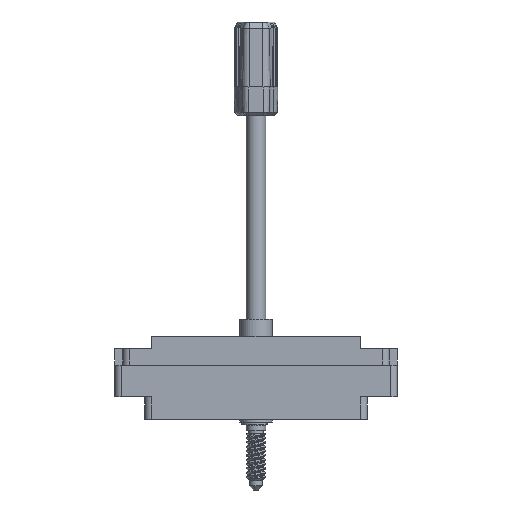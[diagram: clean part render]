
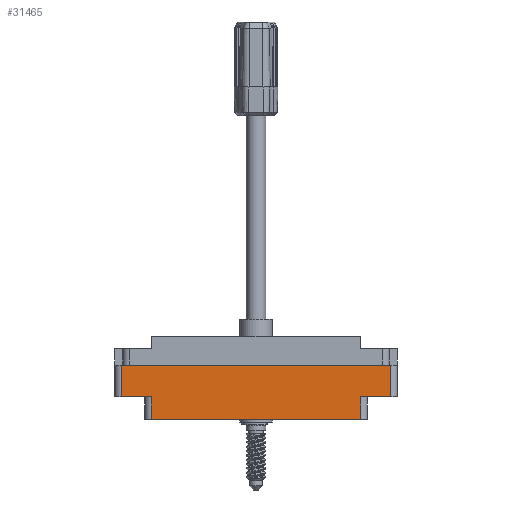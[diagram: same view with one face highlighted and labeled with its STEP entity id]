
A CAD part, front view. The second image highlights one B-rep face of the part: STEP entity #31465.
In plain terms, the highlighted planar face has unit normal (0, -1, 0).
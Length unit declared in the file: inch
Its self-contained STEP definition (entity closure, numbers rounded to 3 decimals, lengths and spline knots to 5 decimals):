
#426 = VERTEX_POINT ( 'NONE', #4976 ) ;
#4279 = VERTEX_POINT ( 'NONE', #10508 ) ;
#4976 = CARTESIAN_POINT ( 'NONE',  ( -1.297, -0.617, -0.274 ) ) ;
#5175 = VERTEX_POINT ( 'NONE', #20055 ) ;
#5830 = EDGE_CURVE ( 'NONE', #5175, #44853, #7103, .T. ) ;
#6219 = EDGE_CURVE ( 'NONE', #52509, #16943, #56597, .T. ) ;
#7103 = LINE ( 'NONE', #20857, #74675 ) ;
#7505 = EDGE_CURVE ( 'NONE', #44853, #25345, #31571, .T. ) ;
#8414 = LINE ( 'NONE', #32848, #31123 ) ;
#8819 = DIRECTION ( 'NONE',  ( 1., 0., 0. ) ) ;
#10450 = ORIENTED_EDGE ( 'NONE', *, *, #16627, .T. ) ;
#10508 = CARTESIAN_POINT ( 'NONE',  ( 1.006, -0.617, -0.798 ) ) ;
#11033 = CARTESIAN_POINT ( 'NONE',  ( -1.006, -0.617, -0.798 ) ) ;
#12350 = VERTEX_POINT ( 'NONE', #67529 ) ;
#12927 = AXIS2_PLACEMENT_3D ( 'NONE', #25637, #32825, #50704 ) ;
#14526 = EDGE_CURVE ( 'NONE', #426, #5175, #35365, .T. ) ;
#15360 = VECTOR ( 'NONE', #67457, 39.37008 ) ;
#16224 = DIRECTION ( 'NONE',  ( -1., 0., 0. ) ) ;
#16627 = EDGE_CURVE ( 'NONE', #52509, #12350, #61151, .T. ) ;
#16943 = VERTEX_POINT ( 'NONE', #73649 ) ;
#20055 = CARTESIAN_POINT ( 'NONE',  ( -1.297, -0.617, -0.578 ) ) ;
#20857 = CARTESIAN_POINT ( 'NONE',  ( 0., -0.617, -0.578 ) ) ;
#21636 = CARTESIAN_POINT ( 'NONE',  ( -1.006, -0.617, -0.578 ) ) ;
#23807 = ORIENTED_EDGE ( 'NONE', *, *, #5830, .T. ) ;
#25345 = VERTEX_POINT ( 'NONE', #54921 ) ;
#25637 = CARTESIAN_POINT ( 'NONE',  ( -1.359, -0.617, -0.798 ) ) ;
#25781 = VECTOR ( 'NONE', #43219, 39.37008 ) ;
#31115 = LINE ( 'NONE', #63827, #77779 ) ;
#31123 = VECTOR ( 'NONE', #62433, 39.37008 ) ;
#31465 = ADVANCED_FACE ( 'NONE', ( #59532 ), #57100, .T. ) ;
#31571 = LINE ( 'NONE', #11033, #41012 ) ;
#31614 = VECTOR ( 'NONE', #40237, 39.37008 ) ;
#32190 = ORIENTED_EDGE ( 'NONE', *, *, #56970, .T. ) ;
#32825 = DIRECTION ( 'NONE',  ( 0., -1., 0. ) ) ;
#32848 = CARTESIAN_POINT ( 'NONE',  ( 1.006, -0.617, -0.578 ) ) ;
#35365 = LINE ( 'NONE', #55311, #15360 ) ;
#37433 = CARTESIAN_POINT ( 'NONE',  ( 1.297, -0.617, -0.798 ) ) ;
#39258 = DIRECTION ( 'NONE',  ( 1., 0., 0. ) ) ;
#40237 = DIRECTION ( 'NONE',  ( 1., 0., 0. ) ) ;
#41012 = VECTOR ( 'NONE', #65511, 39.37008 ) ;
#43219 = DIRECTION ( 'NONE',  ( 0., 0., 1. ) ) ;
#44853 = VERTEX_POINT ( 'NONE', #21636 ) ;
#46531 = EDGE_CURVE ( 'NONE', #426, #12350, #31115, .T. ) ;
#46781 = CARTESIAN_POINT ( 'NONE',  ( 0., -0.617, -0.578 ) ) ;
#48895 = VECTOR ( 'NONE', #16224, 39.37008 ) ;
#49608 = ORIENTED_EDGE ( 'NONE', *, *, #6219, .F. ) ;
#50704 = DIRECTION ( 'NONE',  ( 0., 0., -1. ) ) ;
#50804 = ORIENTED_EDGE ( 'NONE', *, *, #65364, .T. ) ;
#52509 = VERTEX_POINT ( 'NONE', #53066 ) ;
#53066 = CARTESIAN_POINT ( 'NONE',  ( 1.297, -0.617, -0.578 ) ) ;
#54921 = CARTESIAN_POINT ( 'NONE',  ( -1.006, -0.617, -0.798 ) ) ;
#55311 = CARTESIAN_POINT ( 'NONE',  ( -1.297, -0.617, -0.798 ) ) ;
#55640 = ORIENTED_EDGE ( 'NONE', *, *, #14526, .T. ) ;
#56597 = LINE ( 'NONE', #46781, #48895 ) ;
#56970 = EDGE_CURVE ( 'NONE', #4279, #16943, #8414, .T. ) ;
#57100 = PLANE ( 'NONE',  #12927 ) ;
#59532 = FACE_OUTER_BOUND ( 'NONE', #67108, .T. ) ;
#61151 = LINE ( 'NONE', #37433, #25781 ) ;
#61152 = LINE ( 'NONE', #69744, #31614 ) ;
#62433 = DIRECTION ( 'NONE',  ( 0., 0., 1. ) ) ;
#63827 = CARTESIAN_POINT ( 'NONE',  ( 0., -0.617, -0.274 ) ) ;
#65364 = EDGE_CURVE ( 'NONE', #25345, #4279, #61152, .T. ) ;
#65511 = DIRECTION ( 'NONE',  ( 0., 0., -1. ) ) ;
#66785 = ORIENTED_EDGE ( 'NONE', *, *, #46531, .F. ) ;
#67108 = EDGE_LOOP ( 'NONE', ( #23807, #77131, #50804, #32190, #49608, #10450, #66785, #55640 ) ) ;
#67457 = DIRECTION ( 'NONE',  ( 0., 0., -1. ) ) ;
#67529 = CARTESIAN_POINT ( 'NONE',  ( 1.297, -0.617, -0.274 ) ) ;
#69744 = CARTESIAN_POINT ( 'NONE',  ( -1.359, -0.617, -0.798 ) ) ;
#73649 = CARTESIAN_POINT ( 'NONE',  ( 1.006, -0.617, -0.578 ) ) ;
#74675 = VECTOR ( 'NONE', #39258, 39.37008 ) ;
#77131 = ORIENTED_EDGE ( 'NONE', *, *, #7505, .T. ) ;
#77779 = VECTOR ( 'NONE', #8819, 39.37008 ) ;
